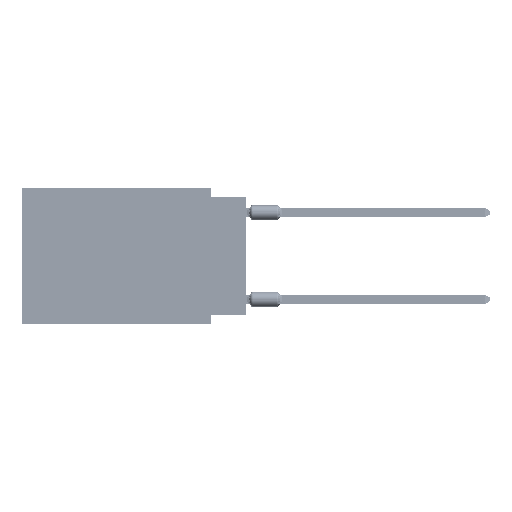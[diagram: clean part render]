
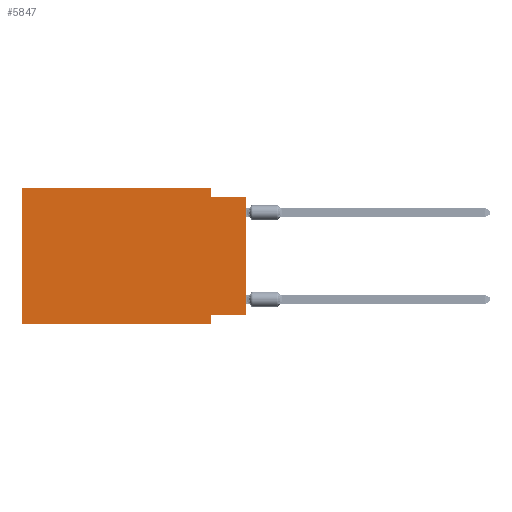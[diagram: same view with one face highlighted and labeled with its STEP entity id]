
A CAD part, left-side view. The second image highlights one B-rep face of the part: STEP entity #5847.
In plain terms, the highlighted planar face has unit normal (-1, 0, 0).
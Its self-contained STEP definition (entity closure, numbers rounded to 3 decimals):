
#2658 = EDGE_LOOP ( 'NONE', ( #80318, #62436, #5610, #16185, #57327, #74618, #20053, #32947 ) ) ;
#3033 = DIRECTION ( 'NONE',  ( 0., 0., 1. ) ) ;
#3385 = EDGE_CURVE ( 'NONE', #70223, #57208, #48338, .T. ) ;
#5610 = ORIENTED_EDGE ( 'NONE', *, *, #74649, .F. ) ;
#5847 = ADVANCED_FACE ( 'NONE', ( #12237 ), #31557, .F. ) ;
#5862 = EDGE_CURVE ( 'NONE', #54406, #57208, #45850, .T. ) ;
#6146 = CARTESIAN_POINT ( 'NONE',  ( 0., 0., -0.635 ) ) ;
#6267 = CARTESIAN_POINT ( 'NONE',  ( 0., 2.54, -0.635 ) ) ;
#7940 = VERTEX_POINT ( 'NONE', #6146 ) ;
#8828 = CARTESIAN_POINT ( 'NONE',  ( 0., 16.383, 0. ) ) ;
#12044 = VERTEX_POINT ( 'NONE', #78001 ) ;
#12088 = CARTESIAN_POINT ( 'NONE',  ( 0., 2.54, -9.271 ) ) ;
#12237 = FACE_OUTER_BOUND ( 'NONE', #2658, .T. ) ;
#12685 = VECTOR ( 'NONE', #64734, 1000. ) ;
#13992 = EDGE_CURVE ( 'NONE', #41786, #7940, #17253, .T. ) ;
#14384 = EDGE_CURVE ( 'NONE', #54406, #18219, #21839, .T. ) ;
#16185 = ORIENTED_EDGE ( 'NONE', *, *, #68421, .F. ) ;
#17253 = LINE ( 'NONE', #74832, #62344 ) ;
#18219 = VERTEX_POINT ( 'NONE', #22169 ) ;
#19292 = DIRECTION ( 'NONE',  ( 0., 1., 0. ) ) ;
#20053 = ORIENTED_EDGE ( 'NONE', *, *, #3385, .F. ) ;
#21839 = LINE ( 'NONE', #8828, #12685 ) ;
#22169 = CARTESIAN_POINT ( 'NONE',  ( 0., 16.383, 0. ) ) ;
#22201 = VECTOR ( 'NONE', #61746, 1000. ) ;
#22235 = VECTOR ( 'NONE', #73569, 1000. ) ;
#22303 = LINE ( 'NONE', #66872, #22235 ) ;
#26047 = DIRECTION ( 'NONE',  ( 0., -1., 0. ) ) ;
#26939 = DIRECTION ( 'NONE',  ( 1., 0., 0. ) ) ;
#31557 = PLANE ( 'NONE',  #57107 ) ;
#31842 = CARTESIAN_POINT ( 'NONE',  ( 0., 16.383, 0. ) ) ;
#32947 = ORIENTED_EDGE ( 'NONE', *, *, #81971, .F. ) ;
#37872 = DIRECTION ( 'NONE',  ( 0., -1., 0. ) ) ;
#41786 = VERTEX_POINT ( 'NONE', #55187 ) ;
#42826 = CARTESIAN_POINT ( 'NONE',  ( 0., 2.54, -9.906 ) ) ;
#45850 = LINE ( 'NONE', #58876, #73247 ) ;
#48338 = LINE ( 'NONE', #42826, #22201 ) ;
#50399 = VECTOR ( 'NONE', #56655, 1000. ) ;
#54406 = VERTEX_POINT ( 'NONE', #54594 ) ;
#54594 = CARTESIAN_POINT ( 'NONE',  ( 0., 16.383, -9.906 ) ) ;
#55187 = CARTESIAN_POINT ( 'NONE',  ( 0., 0., -9.271 ) ) ;
#56631 = VECTOR ( 'NONE', #26047, 1000. ) ;
#56655 = DIRECTION ( 'NONE',  ( 0., -1., 0. ) ) ;
#57107 = AXIS2_PLACEMENT_3D ( 'NONE', #78194, #26939, #70224 ) ;
#57208 = VERTEX_POINT ( 'NONE', #65623 ) ;
#57327 = ORIENTED_EDGE ( 'NONE', *, *, #14384, .F. ) ;
#58404 = LINE ( 'NONE', #71424, #76698 ) ;
#58876 = CARTESIAN_POINT ( 'NONE',  ( 0., 16.383, -9.906 ) ) ;
#61746 = DIRECTION ( 'NONE',  ( 0., 0., -1. ) ) ;
#62344 = VECTOR ( 'NONE', #3033, 1000. ) ;
#62436 = ORIENTED_EDGE ( 'NONE', *, *, #81967, .F. ) ;
#64734 = DIRECTION ( 'NONE',  ( 0., 0., 1. ) ) ;
#65623 = CARTESIAN_POINT ( 'NONE',  ( 0., 2.54, -9.906 ) ) ;
#66872 = CARTESIAN_POINT ( 'NONE',  ( 0., 2.54, 0. ) ) ;
#68421 = EDGE_CURVE ( 'NONE', #18219, #12044, #75556, .T. ) ;
#70223 = VERTEX_POINT ( 'NONE', #12088 ) ;
#70224 = DIRECTION ( 'NONE',  ( 0., 0., -1. ) ) ;
#70583 = LINE ( 'NONE', #77294, #56631 ) ;
#71424 = CARTESIAN_POINT ( 'NONE',  ( 0., 0., -9.271 ) ) ;
#73247 = VECTOR ( 'NONE', #37872, 1000. ) ;
#73569 = DIRECTION ( 'NONE',  ( 0., 0., -1. ) ) ;
#74618 = ORIENTED_EDGE ( 'NONE', *, *, #5862, .T. ) ;
#74649 = EDGE_CURVE ( 'NONE', #12044, #79649, #22303, .T. ) ;
#74832 = CARTESIAN_POINT ( 'NONE',  ( 0., 0., 0. ) ) ;
#75556 = LINE ( 'NONE', #31842, #50399 ) ;
#76698 = VECTOR ( 'NONE', #19292, 1000. ) ;
#77294 = CARTESIAN_POINT ( 'NONE',  ( 0., 0., -0.635 ) ) ;
#78001 = CARTESIAN_POINT ( 'NONE',  ( 0., 2.54, 0. ) ) ;
#78194 = CARTESIAN_POINT ( 'NONE',  ( 0., 16.383, 0. ) ) ;
#79649 = VERTEX_POINT ( 'NONE', #6267 ) ;
#80318 = ORIENTED_EDGE ( 'NONE', *, *, #13992, .T. ) ;
#81967 = EDGE_CURVE ( 'NONE', #79649, #7940, #70583, .T. ) ;
#81971 = EDGE_CURVE ( 'NONE', #41786, #70223, #58404, .T. ) ;
